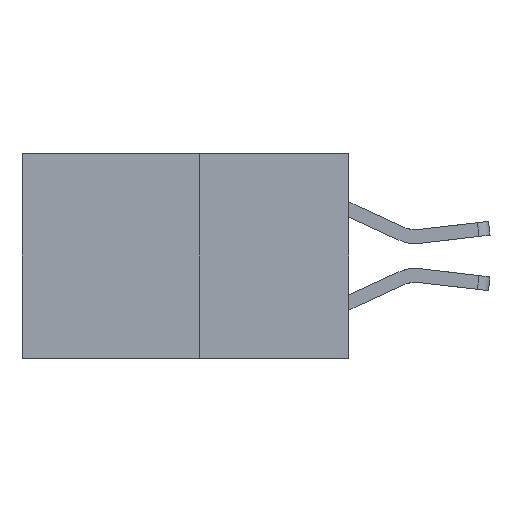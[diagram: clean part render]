
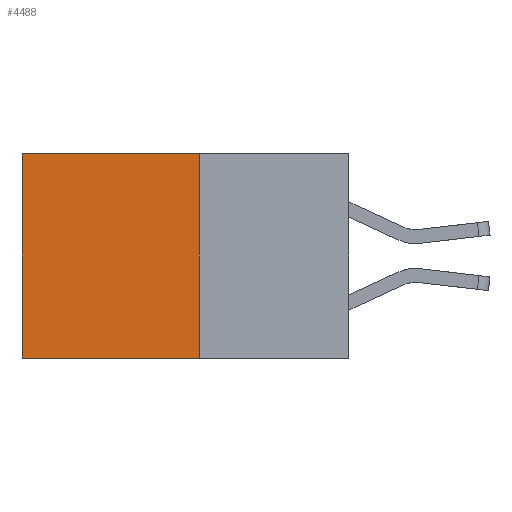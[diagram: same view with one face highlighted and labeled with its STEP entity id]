
A CAD part, left-side view. The second image highlights one B-rep face of the part: STEP entity #4488.
In plain terms, the highlighted planar face has unit normal (-1, 0, 0).
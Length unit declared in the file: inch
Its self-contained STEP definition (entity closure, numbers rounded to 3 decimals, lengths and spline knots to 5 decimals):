
#400 = VECTOR ( 'NONE', #4870, 39.37008 ) ;
#610 = VECTOR ( 'NONE', #1257, 39.37008 ) ;
#668 = CARTESIAN_POINT ( 'NONE',  ( 0.277, 0.27, 0. ) ) ;
#901 = ORIENTED_EDGE ( 'NONE', *, *, #4228, .T. ) ;
#1257 = DIRECTION ( 'NONE',  ( 0., 1., 0. ) ) ;
#1829 = VERTEX_POINT ( 'NONE', #4927 ) ;
#2273 = DIRECTION ( 'NONE',  ( 0., 0., -1. ) ) ;
#2315 = CARTESIAN_POINT ( 'NONE',  ( 0.277, 0.59, -0.37 ) ) ;
#2467 = VECTOR ( 'NONE', #5469, 39.37008 ) ;
#2596 = VERTEX_POINT ( 'NONE', #8577 ) ;
#3028 = AXIS2_PLACEMENT_3D ( 'NONE', #6465, #6404, #6355 ) ;
#3127 = ORIENTED_EDGE ( 'NONE', *, *, #10811, .F. ) ;
#3722 = LINE ( 'NONE', #668, #610 ) ;
#4228 = EDGE_CURVE ( 'NONE', #7498, #2596, #3722, .T. ) ;
#4488 = ADVANCED_FACE ( 'NONE', ( #11630 ), #6681, .F. ) ;
#4870 = DIRECTION ( 'NONE',  ( 0., 0., -1. ) ) ;
#4927 = CARTESIAN_POINT ( 'NONE',  ( 0.277, 0.59, -0.37 ) ) ;
#5349 = CARTESIAN_POINT ( 'NONE',  ( 0.277, 0.27, -0.37 ) ) ;
#5469 = DIRECTION ( 'NONE',  ( 0., 1., 0. ) ) ;
#5506 = ORIENTED_EDGE ( 'NONE', *, *, #9582, .T. ) ;
#5509 = CARTESIAN_POINT ( 'NONE',  ( 0.277, 0.27, -0.37 ) ) ;
#5846 = LINE ( 'NONE', #9344, #400 ) ;
#6355 = DIRECTION ( 'NONE',  ( 0., 0., -1. ) ) ;
#6404 = DIRECTION ( 'NONE',  ( 1., 0., 0. ) ) ;
#6465 = CARTESIAN_POINT ( 'NONE',  ( 0.277, 0.27, -0.37 ) ) ;
#6681 = PLANE ( 'NONE',  #3028 ) ;
#7498 = VERTEX_POINT ( 'NONE', #9211 ) ;
#7535 = LINE ( 'NONE', #2315, #9574 ) ;
#8577 = CARTESIAN_POINT ( 'NONE',  ( 0.277, 0.59, 0. ) ) ;
#9041 = EDGE_CURVE ( 'NONE', #11076, #1829, #10123, .T. ) ;
#9211 = CARTESIAN_POINT ( 'NONE',  ( 0.277, 0.27, 0. ) ) ;
#9344 = CARTESIAN_POINT ( 'NONE',  ( 0.277, 0.27, -0.37 ) ) ;
#9574 = VECTOR ( 'NONE', #2273, 39.37008 ) ;
#9582 = EDGE_CURVE ( 'NONE', #2596, #1829, #7535, .T. ) ;
#10123 = LINE ( 'NONE', #5509, #2467 ) ;
#10166 = ORIENTED_EDGE ( 'NONE', *, *, #9041, .F. ) ;
#10811 = EDGE_CURVE ( 'NONE', #7498, #11076, #5846, .T. ) ;
#10889 = EDGE_LOOP ( 'NONE', ( #5506, #10166, #3127, #901 ) ) ;
#11076 = VERTEX_POINT ( 'NONE', #5349 ) ;
#11630 = FACE_OUTER_BOUND ( 'NONE', #10889, .T. ) ;
